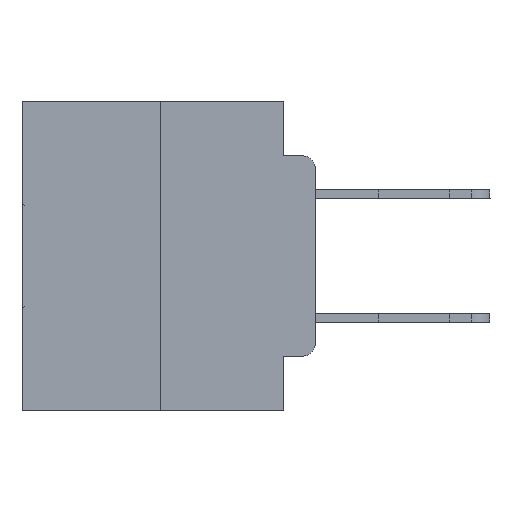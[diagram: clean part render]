
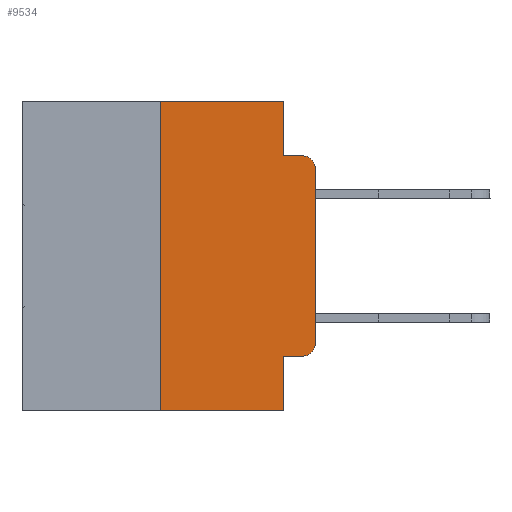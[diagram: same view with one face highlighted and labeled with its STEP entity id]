
A CAD part, left-side view. The second image highlights one B-rep face of the part: STEP entity #9534.
In plain terms, the highlighted planar face has unit normal (-1, 0, 0).
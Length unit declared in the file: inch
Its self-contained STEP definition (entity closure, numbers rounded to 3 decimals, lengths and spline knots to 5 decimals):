
#1082 = EDGE_CURVE ( 'NONE', #20691, #29509, #21746, .T. ) ;
#1110 = DIRECTION ( 'NONE',  ( -1., 0., 0. ) ) ;
#1742 = CIRCLE ( 'NONE', #8195, 0.02 ) ;
#1824 = CARTESIAN_POINT ( 'NONE',  ( 0., 0.25, -0.5 ) ) ;
#2272 = CARTESIAN_POINT ( 'NONE',  ( 0., 0.051, 0. ) ) ;
#2411 = ORIENTED_EDGE ( 'NONE', *, *, #21297, .T. ) ;
#2642 = CARTESIAN_POINT ( 'NONE',  ( 0., 0.473, 0. ) ) ;
#3665 = CARTESIAN_POINT ( 'NONE',  ( 0., 0., -0.1085 ) ) ;
#4043 = ORIENTED_EDGE ( 'NONE', *, *, #29189, .F. ) ;
#4723 = CARTESIAN_POINT ( 'NONE',  ( 0., 0.051, -0.0885 ) ) ;
#4800 = ORIENTED_EDGE ( 'NONE', *, *, #24440, .F. ) ;
#5027 = CARTESIAN_POINT ( 'NONE',  ( 0., 0.25, 0. ) ) ;
#5058 = DIRECTION ( 'NONE',  ( 0., 0., -1. ) ) ;
#5660 = VERTEX_POINT ( 'NONE', #24789 ) ;
#5756 = CARTESIAN_POINT ( 'NONE',  ( 0., 0., 0. ) ) ;
#6031 = EDGE_CURVE ( 'NONE', #6482, #29509, #1742, .T. ) ;
#6063 = LINE ( 'NONE', #7007, #11889 ) ;
#6183 = ORIENTED_EDGE ( 'NONE', *, *, #1082, .F. ) ;
#6409 = DIRECTION ( 'NONE',  ( 0., -1., 0. ) ) ;
#6482 = VERTEX_POINT ( 'NONE', #3665 ) ;
#7007 = CARTESIAN_POINT ( 'NONE',  ( 0., 0.473, 0. ) ) ;
#7137 = VERTEX_POINT ( 'NONE', #22966 ) ;
#7701 = EDGE_CURVE ( 'NONE', #17513, #6482, #12073, .T. ) ;
#7767 = CARTESIAN_POINT ( 'NONE',  ( 0., 0.051, -0.4115 ) ) ;
#7828 = DIRECTION ( 'NONE',  ( 0., -1., 0. ) ) ;
#8195 = AXIS2_PLACEMENT_3D ( 'NONE', #14263, #30835, #16670 ) ;
#8238 = VECTOR ( 'NONE', #21567, 39.37008 ) ;
#8299 = DIRECTION ( 'NONE',  ( 0., 0., 1. ) ) ;
#8428 = VERTEX_POINT ( 'NONE', #20410 ) ;
#8788 = CARTESIAN_POINT ( 'NONE',  ( 0., 0.02, -0.0885 ) ) ;
#9534 = ADVANCED_FACE ( 'NONE', ( #25502 ), #10043, .F. ) ;
#9723 = AXIS2_PLACEMENT_3D ( 'NONE', #2642, #19691, #5058 ) ;
#9738 = VECTOR ( 'NONE', #7828, 39.37008 ) ;
#9851 = VERTEX_POINT ( 'NONE', #30102 ) ;
#10043 = PLANE ( 'NONE',  #9723 ) ;
#11889 = VECTOR ( 'NONE', #21533, 39.37008 ) ;
#12073 = LINE ( 'NONE', #5756, #30281 ) ;
#12407 = ORIENTED_EDGE ( 'NONE', *, *, #26432, .T. ) ;
#12533 = EDGE_CURVE ( 'NONE', #9851, #7137, #6063, .T. ) ;
#13153 = LINE ( 'NONE', #2272, #30601 ) ;
#13768 = ORIENTED_EDGE ( 'NONE', *, *, #6031, .T. ) ;
#14263 = CARTESIAN_POINT ( 'NONE',  ( 0., 0.02, -0.1085 ) ) ;
#15630 = CARTESIAN_POINT ( 'NONE',  ( 0., 0.051, -0.0885 ) ) ;
#15809 = CARTESIAN_POINT ( 'NONE',  ( 0., 0.02, -0.3915 ) ) ;
#16143 = CARTESIAN_POINT ( 'NONE',  ( 0., 0.473, -0.5 ) ) ;
#16449 = CARTESIAN_POINT ( 'NONE',  ( 0., 0.051, 0. ) ) ;
#16670 = DIRECTION ( 'NONE',  ( 0., 0., -1. ) ) ;
#17513 = VERTEX_POINT ( 'NONE', #28038 ) ;
#17844 = VECTOR ( 'NONE', #18832, 39.37008 ) ;
#17891 = VERTEX_POINT ( 'NONE', #7767 ) ;
#17901 = LINE ( 'NONE', #5027, #18638 ) ;
#18216 = DIRECTION ( 'NONE',  ( 0., 0., -1. ) ) ;
#18638 = VECTOR ( 'NONE', #22041, 39.37008 ) ;
#18832 = DIRECTION ( 'NONE',  ( 0., 0., -1. ) ) ;
#19163 = CARTESIAN_POINT ( 'NONE',  ( 0., 0.051, -0.4115 ) ) ;
#19387 = ORIENTED_EDGE ( 'NONE', *, *, #22876, .T. ) ;
#19691 = DIRECTION ( 'NONE',  ( 1., 0., 0. ) ) ;
#20002 = ORIENTED_EDGE ( 'NONE', *, *, #12533, .F. ) ;
#20410 = CARTESIAN_POINT ( 'NONE',  ( 0., 0.02, -0.4115 ) ) ;
#20691 = VERTEX_POINT ( 'NONE', #15630 ) ;
#20855 = LINE ( 'NONE', #16449, #17844 ) ;
#21002 = ORIENTED_EDGE ( 'NONE', *, *, #30764, .F. ) ;
#21089 = LINE ( 'NONE', #19163, #8238 ) ;
#21297 = EDGE_CURVE ( 'NONE', #8428, #17513, #26341, .T. ) ;
#21533 = DIRECTION ( 'NONE',  ( 0., -1., 0. ) ) ;
#21567 = DIRECTION ( 'NONE',  ( 0., -1., 0. ) ) ;
#21746 = LINE ( 'NONE', #4723, #9738 ) ;
#22041 = DIRECTION ( 'NONE',  ( 0., 0., 1. ) ) ;
#22550 = VECTOR ( 'NONE', #6409, 39.37008 ) ;
#22876 = EDGE_CURVE ( 'NONE', #17891, #8428, #21089, .T. ) ;
#22966 = CARTESIAN_POINT ( 'NONE',  ( 0., 0.051, 0. ) ) ;
#24440 = EDGE_CURVE ( 'NONE', #17891, #5660, #13153, .T. ) ;
#24789 = CARTESIAN_POINT ( 'NONE',  ( 0., 0.051, -0.5 ) ) ;
#25502 = FACE_OUTER_BOUND ( 'NONE', #28607, .T. ) ;
#26341 = CIRCLE ( 'NONE', #29273, 0.02 ) ;
#26432 = EDGE_CURVE ( 'NONE', #29663, #5660, #28838, .T. ) ;
#28038 = CARTESIAN_POINT ( 'NONE',  ( 0., 0., -0.3915 ) ) ;
#28607 = EDGE_LOOP ( 'NONE', ( #28615, #13768, #6183, #21002, #20002, #4043, #12407, #4800, #19387, #2411 ) ) ;
#28615 = ORIENTED_EDGE ( 'NONE', *, *, #7701, .T. ) ;
#28838 = LINE ( 'NONE', #16143, #22550 ) ;
#29189 = EDGE_CURVE ( 'NONE', #29663, #9851, #17901, .T. ) ;
#29273 = AXIS2_PLACEMENT_3D ( 'NONE', #15809, #1110, #18216 ) ;
#29509 = VERTEX_POINT ( 'NONE', #8788 ) ;
#29663 = VERTEX_POINT ( 'NONE', #1824 ) ;
#30102 = CARTESIAN_POINT ( 'NONE',  ( 0., 0.25, 0. ) ) ;
#30281 = VECTOR ( 'NONE', #8299, 39.37008 ) ;
#30601 = VECTOR ( 'NONE', #31091, 39.37008 ) ;
#30764 = EDGE_CURVE ( 'NONE', #7137, #20691, #20855, .T. ) ;
#30835 = DIRECTION ( 'NONE',  ( -1., 0., 0. ) ) ;
#31091 = DIRECTION ( 'NONE',  ( 0., 0., -1. ) ) ;
